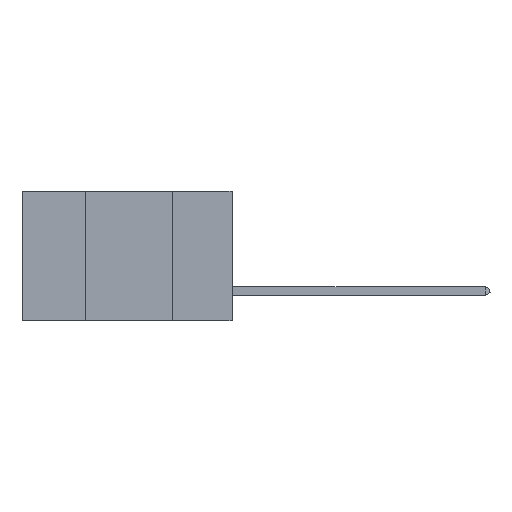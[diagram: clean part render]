
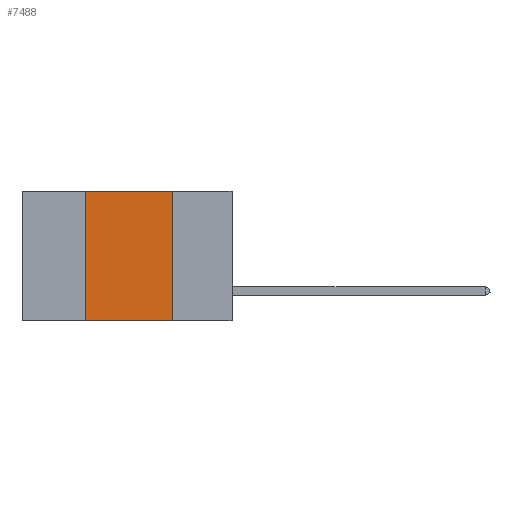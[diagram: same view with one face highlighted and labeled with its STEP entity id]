
A CAD part, left-side view. The second image highlights one B-rep face of the part: STEP entity #7488.
In plain terms, the highlighted planar face has unit normal (-1, 0, 0).
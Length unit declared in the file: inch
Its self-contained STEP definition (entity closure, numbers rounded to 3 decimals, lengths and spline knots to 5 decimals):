
#58 = LINE ( 'NONE', #3821, #9116 ) ;
#653 = DIRECTION ( 'NONE',  ( 0., 0., 1. ) ) ;
#850 = VERTEX_POINT ( 'NONE', #8421 ) ;
#1213 = FACE_OUTER_BOUND ( 'NONE', #1411, .T. ) ;
#1334 = DIRECTION ( 'NONE',  ( 1., 0., 0. ) ) ;
#1357 = DIRECTION ( 'NONE',  ( 0., 0., -1. ) ) ;
#1411 = EDGE_LOOP ( 'NONE', ( #4057, #1839, #4903, #1869 ) ) ;
#1736 = LINE ( 'NONE', #8141, #5384 ) ;
#1839 = ORIENTED_EDGE ( 'NONE', *, *, #9276, .F. ) ;
#1869 = ORIENTED_EDGE ( 'NONE', *, *, #10871, .T. ) ;
#2556 = CARTESIAN_POINT ( 'NONE',  ( 0., 0.6, 0. ) ) ;
#2863 = VERTEX_POINT ( 'NONE', #9250 ) ;
#3821 = CARTESIAN_POINT ( 'NONE',  ( 0., 0.17, 0. ) ) ;
#3931 = VECTOR ( 'NONE', #653, 39.37008 ) ;
#4057 = ORIENTED_EDGE ( 'NONE', *, *, #8401, .F. ) ;
#4062 = CARTESIAN_POINT ( 'NONE',  ( 0., 0.6, 0. ) ) ;
#4903 = ORIENTED_EDGE ( 'NONE', *, *, #5946, .F. ) ;
#5014 = AXIS2_PLACEMENT_3D ( 'NONE', #4062, #1334, #8427 ) ;
#5138 = CARTESIAN_POINT ( 'NONE',  ( 0., 0.42, 0. ) ) ;
#5253 = DIRECTION ( 'NONE',  ( 0., -1., 0. ) ) ;
#5384 = VECTOR ( 'NONE', #7261, 39.37008 ) ;
#5946 = EDGE_CURVE ( 'NONE', #11051, #6928, #6628, .T. ) ;
#6628 = LINE ( 'NONE', #5138, #3931 ) ;
#6928 = VERTEX_POINT ( 'NONE', #11620 ) ;
#7136 = VECTOR ( 'NONE', #5253, 39.37008 ) ;
#7261 = DIRECTION ( 'NONE',  ( 0., -1., 0. ) ) ;
#7488 = ADVANCED_FACE ( 'NONE', ( #1213 ), #11283, .F. ) ;
#8141 = CARTESIAN_POINT ( 'NONE',  ( 0., 0.6, -0.37 ) ) ;
#8401 = EDGE_CURVE ( 'NONE', #850, #2863, #58, .T. ) ;
#8421 = CARTESIAN_POINT ( 'NONE',  ( 0., 0.17, 0. ) ) ;
#8427 = DIRECTION ( 'NONE',  ( 0., 0., -1. ) ) ;
#9116 = VECTOR ( 'NONE', #1357, 39.37008 ) ;
#9250 = CARTESIAN_POINT ( 'NONE',  ( 0., 0.17, -0.37 ) ) ;
#9276 = EDGE_CURVE ( 'NONE', #6928, #850, #9560, .T. ) ;
#9523 = CARTESIAN_POINT ( 'NONE',  ( 0., 0.42, -0.37 ) ) ;
#9560 = LINE ( 'NONE', #2556, #7136 ) ;
#10871 = EDGE_CURVE ( 'NONE', #11051, #2863, #1736, .T. ) ;
#11051 = VERTEX_POINT ( 'NONE', #9523 ) ;
#11283 = PLANE ( 'NONE',  #5014 ) ;
#11620 = CARTESIAN_POINT ( 'NONE',  ( 0., 0.42, 0. ) ) ;
